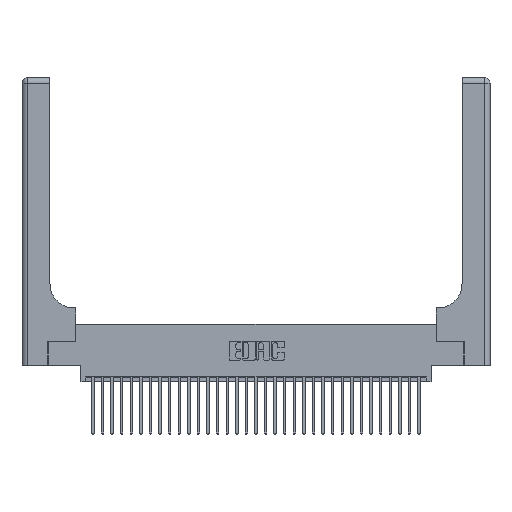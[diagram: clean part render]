
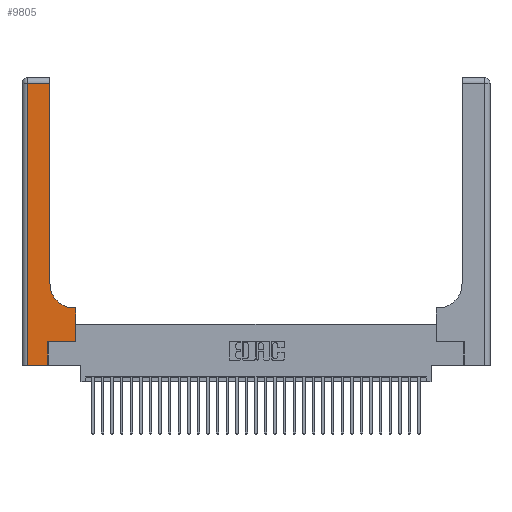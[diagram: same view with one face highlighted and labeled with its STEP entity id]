
A CAD part, top view. The second image highlights one B-rep face of the part: STEP entity #9805.
In plain terms, the highlighted planar face has unit normal (0, 0, 1).
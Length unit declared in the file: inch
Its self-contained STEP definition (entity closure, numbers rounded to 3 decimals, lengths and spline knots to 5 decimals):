
#1520 = PLANE ( 'NONE',  #8907 ) ;
#1724 = EDGE_CURVE ( 'NONE', #18477, #13858, #23064, .T. ) ;
#1733 = DIRECTION ( 'NONE',  ( 0., 1., 0. ) ) ;
#1850 = DIRECTION ( 'NONE',  ( -1., 0., 0. ) ) ;
#2304 = CARTESIAN_POINT ( 'NONE',  ( 0.269, 0., 0.37 ) ) ;
#2495 = VERTEX_POINT ( 'NONE', #2304 ) ;
#2665 = CARTESIAN_POINT ( 'NONE',  ( 0.269, 0.25, 0.37 ) ) ;
#2759 = EDGE_LOOP ( 'NONE', ( #6827, #24880, #22898, #16160, #29901, #23956, #32742, #26121, #20310 ) ) ;
#3052 = EDGE_CURVE ( 'NONE', #2495, #32306, #26317, .T. ) ;
#3528 = EDGE_CURVE ( 'NONE', #15286, #7231, #31145, .T. ) ;
#3536 = CARTESIAN_POINT ( 'NONE',  ( 0.5585, 0.25, 0.37 ) ) ;
#5562 = EDGE_CURVE ( 'NONE', #7231, #29699, #19224, .T. ) ;
#5714 = DIRECTION ( 'NONE',  ( 0., -1., 0. ) ) ;
#5943 = FACE_OUTER_BOUND ( 'NONE', #2759, .T. ) ;
#6226 = LINE ( 'NONE', #16035, #16386 ) ;
#6827 = ORIENTED_EDGE ( 'NONE', *, *, #3528, .T. ) ;
#7231 = VERTEX_POINT ( 'NONE', #21218 ) ;
#7423 = CARTESIAN_POINT ( 'NONE',  ( 0.5415, 0.6, 0.37 ) ) ;
#8907 = AXIS2_PLACEMENT_3D ( 'NONE', #32874, #30465, #1850 ) ;
#9116 = VECTOR ( 'NONE', #30993, 39.37008 ) ;
#9805 = ADVANCED_FACE ( 'NONE', ( #5943 ), #1520, .F. ) ;
#10948 = EDGE_CURVE ( 'NONE', #29699, #18050, #6226, .T. ) ;
#11208 = DIRECTION ( 'NONE',  ( 0., 0., -1. ) ) ;
#11777 = LINE ( 'NONE', #22396, #20363 ) ;
#12151 = DIRECTION ( 'NONE',  ( 1., 0., 0. ) ) ;
#13848 = EDGE_CURVE ( 'NONE', #18050, #2495, #13963, .T. ) ;
#13858 = VERTEX_POINT ( 'NONE', #7423 ) ;
#13963 = LINE ( 'NONE', #17666, #9116 ) ;
#14103 = CIRCLE ( 'NONE', #22550, 0.25 ) ;
#14302 = CARTESIAN_POINT ( 'NONE',  ( 0.269, 0., 0.37 ) ) ;
#15286 = VERTEX_POINT ( 'NONE', #18537 ) ;
#15491 = EDGE_CURVE ( 'NONE', #21068, #18477, #30600, .T. ) ;
#15522 = CARTESIAN_POINT ( 'NONE',  ( 0.2915, 0.6, 0.37 ) ) ;
#16035 = CARTESIAN_POINT ( 'NONE',  ( 0.06, 3., 0.37 ) ) ;
#16149 = VECTOR ( 'NONE', #25306, 39.37008 ) ;
#16160 = ORIENTED_EDGE ( 'NONE', *, *, #13848, .T. ) ;
#16386 = VECTOR ( 'NONE', #5714, 39.37008 ) ;
#16672 = CARTESIAN_POINT ( 'NONE',  ( 0.5415, 0.85, 0.37 ) ) ;
#17052 = DIRECTION ( 'NONE',  ( 0., 1., 0. ) ) ;
#17352 = CARTESIAN_POINT ( 'NONE',  ( 0.5585, 0.25, 0.37 ) ) ;
#17434 = CARTESIAN_POINT ( 'NONE',  ( 0.06, 2.94, 0.37 ) ) ;
#17530 = EDGE_CURVE ( 'NONE', #13858, #15286, #14103, .T. ) ;
#17666 = CARTESIAN_POINT ( 'NONE',  ( 0., 0., 0.37 ) ) ;
#17951 = VECTOR ( 'NONE', #1733, 39.37008 ) ;
#18050 = VERTEX_POINT ( 'NONE', #26343 ) ;
#18477 = VERTEX_POINT ( 'NONE', #23669 ) ;
#18537 = CARTESIAN_POINT ( 'NONE',  ( 0.2915, 0.85, 0.37 ) ) ;
#19224 = LINE ( 'NONE', #33524, #26957 ) ;
#19390 = VECTOR ( 'NONE', #17052, 39.37008 ) ;
#20310 = ORIENTED_EDGE ( 'NONE', *, *, #17530, .T. ) ;
#20363 = VECTOR ( 'NONE', #12151, 39.37008 ) ;
#21068 = VERTEX_POINT ( 'NONE', #3536 ) ;
#21218 = CARTESIAN_POINT ( 'NONE',  ( 0.2915, 2.94, 0.37 ) ) ;
#22396 = CARTESIAN_POINT ( 'NONE',  ( 0.269, 0.25, 0.37 ) ) ;
#22550 = AXIS2_PLACEMENT_3D ( 'NONE', #16672, #11208, #32288 ) ;
#22898 = ORIENTED_EDGE ( 'NONE', *, *, #10948, .T. ) ;
#23064 = LINE ( 'NONE', #15522, #16149 ) ;
#23669 = CARTESIAN_POINT ( 'NONE',  ( 0.5585, 0.6, 0.37 ) ) ;
#23956 = ORIENTED_EDGE ( 'NONE', *, *, #24618, .T. ) ;
#24618 = EDGE_CURVE ( 'NONE', #32306, #21068, #11777, .T. ) ;
#24880 = ORIENTED_EDGE ( 'NONE', *, *, #5562, .T. ) ;
#25306 = DIRECTION ( 'NONE',  ( -1., 0., 0. ) ) ;
#26121 = ORIENTED_EDGE ( 'NONE', *, *, #1724, .T. ) ;
#26317 = LINE ( 'NONE', #14302, #19390 ) ;
#26343 = CARTESIAN_POINT ( 'NONE',  ( 0.06, 0., 0.37 ) ) ;
#26957 = VECTOR ( 'NONE', #33309, 39.37008 ) ;
#27245 = DIRECTION ( 'NONE',  ( 0., 1., 0. ) ) ;
#29699 = VERTEX_POINT ( 'NONE', #17434 ) ;
#29901 = ORIENTED_EDGE ( 'NONE', *, *, #3052, .T. ) ;
#30465 = DIRECTION ( 'NONE',  ( 0., 0., -1. ) ) ;
#30600 = LINE ( 'NONE', #17352, #17951 ) ;
#30993 = DIRECTION ( 'NONE',  ( 1., 0., 0. ) ) ;
#31145 = LINE ( 'NONE', #32392, #33194 ) ;
#32288 = DIRECTION ( 'NONE',  ( 1., 0., 0. ) ) ;
#32306 = VERTEX_POINT ( 'NONE', #2665 ) ;
#32392 = CARTESIAN_POINT ( 'NONE',  ( 0.2915, 3., 0.37 ) ) ;
#32742 = ORIENTED_EDGE ( 'NONE', *, *, #15491, .T. ) ;
#32874 = CARTESIAN_POINT ( 'NONE',  ( 0., 3., 0.37 ) ) ;
#33194 = VECTOR ( 'NONE', #27245, 39.37008 ) ;
#33309 = DIRECTION ( 'NONE',  ( -1., 0., 0. ) ) ;
#33524 = CARTESIAN_POINT ( 'NONE',  ( 0., 2.94, 0.37 ) ) ;
